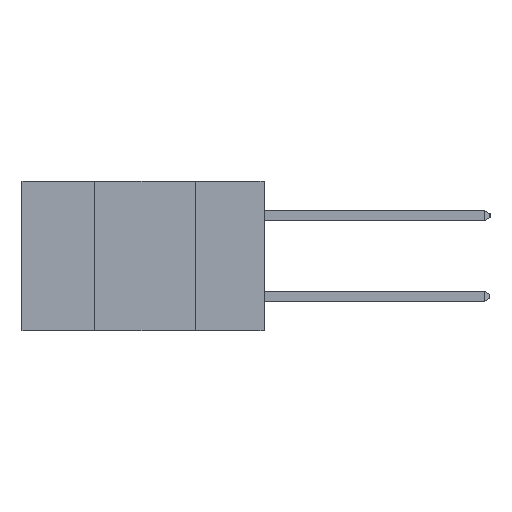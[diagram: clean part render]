
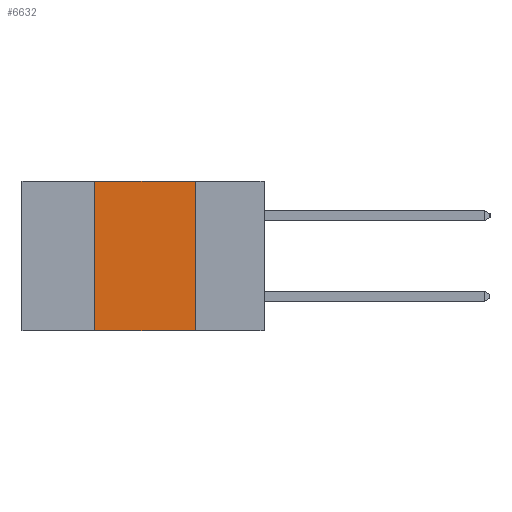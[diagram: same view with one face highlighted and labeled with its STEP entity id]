
A CAD part, left-side view. The second image highlights one B-rep face of the part: STEP entity #6632.
In plain terms, the highlighted planar face has unit normal (-1, 0, 0).
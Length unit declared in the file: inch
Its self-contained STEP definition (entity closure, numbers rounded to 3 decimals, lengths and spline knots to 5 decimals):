
#856 = LINE ( 'NONE', #3638, #14669 ) ;
#1503 = ORIENTED_EDGE ( 'NONE', *, *, #12927, .F. ) ;
#3205 = AXIS2_PLACEMENT_3D ( 'NONE', #16424, #9259, #21708 ) ;
#3445 = CARTESIAN_POINT ( 'NONE',  ( 0., 0.17, -0.37 ) ) ;
#3449 = LINE ( 'NONE', #10263, #12443 ) ;
#3454 = DIRECTION ( 'NONE',  ( 0., 0., -1. ) ) ;
#3638 = CARTESIAN_POINT ( 'NONE',  ( 0., 0.17, -0.37 ) ) ;
#4005 = CARTESIAN_POINT ( 'NONE',  ( 0., 0.6, 0. ) ) ;
#4801 = VERTEX_POINT ( 'NONE', #12681 ) ;
#5244 = EDGE_CURVE ( 'NONE', #15070, #20411, #856, .T. ) ;
#5263 = LINE ( 'NONE', #4005, #14258 ) ;
#5822 = DIRECTION ( 'NONE',  ( 0., -1., 0. ) ) ;
#6632 = ADVANCED_FACE ( 'NONE', ( #14591 ), #18187, .F. ) ;
#6828 = ORIENTED_EDGE ( 'NONE', *, *, #5244, .F. ) ;
#7692 = CARTESIAN_POINT ( 'NONE',  ( 0., 0.42, -0.37 ) ) ;
#9259 = DIRECTION ( 'NONE',  ( 1., 0., 0. ) ) ;
#10263 = CARTESIAN_POINT ( 'NONE',  ( 0., 0.6, -0.37 ) ) ;
#10483 = ORIENTED_EDGE ( 'NONE', *, *, #13934, .T. ) ;
#12085 = DIRECTION ( 'NONE',  ( 0., -1., 0. ) ) ;
#12443 = VECTOR ( 'NONE', #12085, 39.37008 ) ;
#12681 = CARTESIAN_POINT ( 'NONE',  ( 0., 0.42, 0. ) ) ;
#12927 = EDGE_CURVE ( 'NONE', #14936, #4801, #19983, .T. ) ;
#13934 = EDGE_CURVE ( 'NONE', #14936, #20411, #3449, .T. ) ;
#14258 = VECTOR ( 'NONE', #5822, 39.37008 ) ;
#14591 = FACE_OUTER_BOUND ( 'NONE', #15673, .T. ) ;
#14669 = VECTOR ( 'NONE', #3454, 39.37008 ) ;
#14936 = VERTEX_POINT ( 'NONE', #18436 ) ;
#15070 = VERTEX_POINT ( 'NONE', #17166 ) ;
#15673 = EDGE_LOOP ( 'NONE', ( #6828, #20504, #1503, #10483 ) ) ;
#16424 = CARTESIAN_POINT ( 'NONE',  ( 0., 0.6, 0. ) ) ;
#17166 = CARTESIAN_POINT ( 'NONE',  ( 0., 0.17, 0. ) ) ;
#18187 = PLANE ( 'NONE',  #3205 ) ;
#18436 = CARTESIAN_POINT ( 'NONE',  ( 0., 0.42, -0.37 ) ) ;
#19404 = VECTOR ( 'NONE', #21959, 39.37008 ) ;
#19983 = LINE ( 'NONE', #7692, #19404 ) ;
#20411 = VERTEX_POINT ( 'NONE', #3445 ) ;
#20504 = ORIENTED_EDGE ( 'NONE', *, *, #22482, .F. ) ;
#21708 = DIRECTION ( 'NONE',  ( 0., 0., -1. ) ) ;
#21959 = DIRECTION ( 'NONE',  ( 0., 0., 1. ) ) ;
#22482 = EDGE_CURVE ( 'NONE', #4801, #15070, #5263, .T. ) ;
